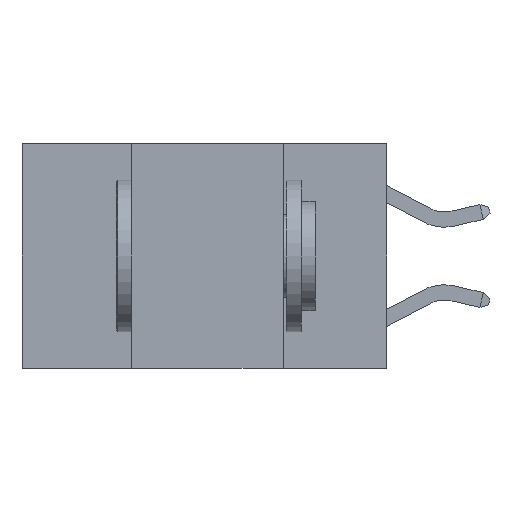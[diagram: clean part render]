
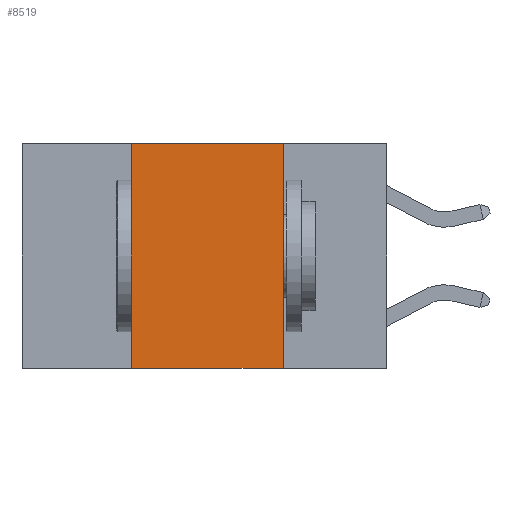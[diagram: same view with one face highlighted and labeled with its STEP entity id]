
A CAD part, left-side view. The second image highlights one B-rep face of the part: STEP entity #8519.
In plain terms, the highlighted planar face has unit normal (-1, 0, 0).
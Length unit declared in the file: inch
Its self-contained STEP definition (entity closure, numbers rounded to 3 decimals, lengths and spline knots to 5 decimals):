
#19 = CARTESIAN_POINT ( 'NONE',  ( 0., 0.17, -0.37 ) ) ;
#70 = EDGE_CURVE ( 'NONE', #5008, #2160, #670, .T. ) ;
#670 = LINE ( 'NONE', #6741, #8497 ) ;
#1215 = ORIENTED_EDGE ( 'NONE', *, *, #9721, .T. ) ;
#1910 = DIRECTION ( 'NONE',  ( 0., 0., -1. ) ) ;
#2041 = ORIENTED_EDGE ( 'NONE', *, *, #4928, .F. ) ;
#2160 = VERTEX_POINT ( 'NONE', #19 ) ;
#2214 = VECTOR ( 'NONE', #2351, 39.37008 ) ;
#2351 = DIRECTION ( 'NONE',  ( 0., 0., 1. ) ) ;
#2505 = VECTOR ( 'NONE', #4901, 39.37008 ) ;
#2875 = FACE_OUTER_BOUND ( 'NONE', #5824, .T. ) ;
#3441 = CARTESIAN_POINT ( 'NONE',  ( 0., 0.42, 0. ) ) ;
#3832 = CARTESIAN_POINT ( 'NONE',  ( 0., 0.42, 0. ) ) ;
#4118 = CARTESIAN_POINT ( 'NONE',  ( 0., 0.6, -0.37 ) ) ;
#4494 = LINE ( 'NONE', #4118, #2505 ) ;
#4557 = CARTESIAN_POINT ( 'NONE',  ( 0., 0.6, 0. ) ) ;
#4861 = VERTEX_POINT ( 'NONE', #8247 ) ;
#4901 = DIRECTION ( 'NONE',  ( 0., -1., 0. ) ) ;
#4928 = EDGE_CURVE ( 'NONE', #6659, #5008, #9099, .T. ) ;
#5008 = VERTEX_POINT ( 'NONE', #6964 ) ;
#5116 = ORIENTED_EDGE ( 'NONE', *, *, #70, .F. ) ;
#5615 = EDGE_CURVE ( 'NONE', #4861, #6659, #6245, .T. ) ;
#5824 = EDGE_LOOP ( 'NONE', ( #5116, #2041, #9591, #1215 ) ) ;
#6245 = LINE ( 'NONE', #3832, #2214 ) ;
#6350 = DIRECTION ( 'NONE',  ( 0., 0., -1. ) ) ;
#6469 = DIRECTION ( 'NONE',  ( 1., 0., 0. ) ) ;
#6541 = AXIS2_PLACEMENT_3D ( 'NONE', #8678, #6469, #1910 ) ;
#6659 = VERTEX_POINT ( 'NONE', #3441 ) ;
#6741 = CARTESIAN_POINT ( 'NONE',  ( 0., 0.17, 0. ) ) ;
#6906 = VECTOR ( 'NONE', #8317, 39.37008 ) ;
#6964 = CARTESIAN_POINT ( 'NONE',  ( 0., 0.17, 0. ) ) ;
#7927 = PLANE ( 'NONE',  #6541 ) ;
#8247 = CARTESIAN_POINT ( 'NONE',  ( 0., 0.42, -0.37 ) ) ;
#8317 = DIRECTION ( 'NONE',  ( 0., -1., 0. ) ) ;
#8497 = VECTOR ( 'NONE', #6350, 39.37008 ) ;
#8519 = ADVANCED_FACE ( 'NONE', ( #2875 ), #7927, .F. ) ;
#8678 = CARTESIAN_POINT ( 'NONE',  ( 0., 0.6, 0. ) ) ;
#9099 = LINE ( 'NONE', #4557, #6906 ) ;
#9591 = ORIENTED_EDGE ( 'NONE', *, *, #5615, .F. ) ;
#9721 = EDGE_CURVE ( 'NONE', #4861, #2160, #4494, .T. ) ;
